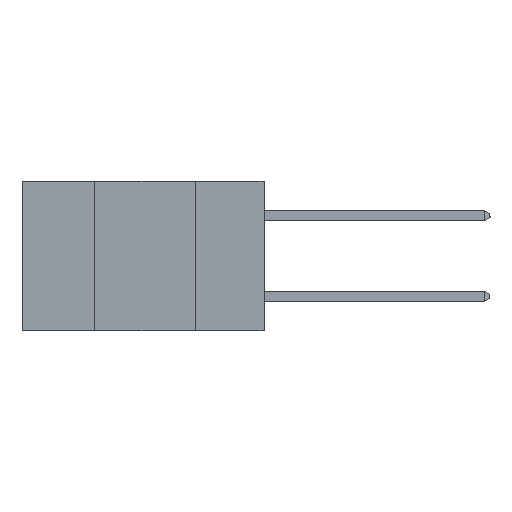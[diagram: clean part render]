
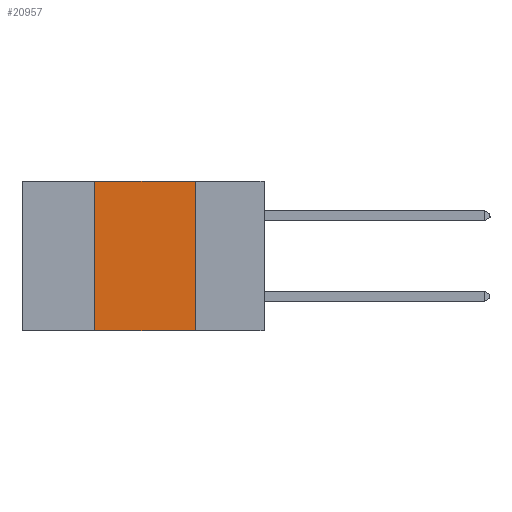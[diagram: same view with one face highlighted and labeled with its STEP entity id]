
A CAD part, left-side view. The second image highlights one B-rep face of the part: STEP entity #20957.
In plain terms, the highlighted planar face has unit normal (-1, 0, 0).
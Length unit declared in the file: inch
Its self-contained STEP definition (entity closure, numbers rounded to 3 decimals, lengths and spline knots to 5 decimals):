
#307 = VERTEX_POINT ( 'NONE', #8953 ) ;
#450 = ORIENTED_EDGE ( 'NONE', *, *, #4845, .F. ) ;
#1586 = AXIS2_PLACEMENT_3D ( 'NONE', #9550, #26071, #13766 ) ;
#1791 = LINE ( 'NONE', #19559, #22508 ) ;
#2050 = LINE ( 'NONE', #19369, #16722 ) ;
#4401 = FACE_OUTER_BOUND ( 'NONE', #11159, .T. ) ;
#4845 = EDGE_CURVE ( 'NONE', #18505, #307, #6566, .T. ) ;
#5902 = DIRECTION ( 'NONE',  ( 0., 0., 1. ) ) ;
#6032 = CARTESIAN_POINT ( 'NONE',  ( 0., 0.17, -0.37 ) ) ;
#6363 = CARTESIAN_POINT ( 'NONE',  ( 0., 0.42, -0.37 ) ) ;
#6566 = LINE ( 'NONE', #16216, #22430 ) ;
#8953 = CARTESIAN_POINT ( 'NONE',  ( 0., 0.42, 0. ) ) ;
#9463 = VECTOR ( 'NONE', #15052, 39.37008 ) ;
#9550 = CARTESIAN_POINT ( 'NONE',  ( 0., 0.6, 0. ) ) ;
#11159 = EDGE_LOOP ( 'NONE', ( #15808, #21858, #450, #11524 ) ) ;
#11524 = ORIENTED_EDGE ( 'NONE', *, *, #17926, .T. ) ;
#12792 = VERTEX_POINT ( 'NONE', #26674 ) ;
#12945 = CARTESIAN_POINT ( 'NONE',  ( 0., 0.6, -0.37 ) ) ;
#13123 = EDGE_CURVE ( 'NONE', #307, #12792, #2050, .T. ) ;
#13457 = DIRECTION ( 'NONE',  ( 0., 0., -1. ) ) ;
#13766 = DIRECTION ( 'NONE',  ( 0., 0., -1. ) ) ;
#15052 = DIRECTION ( 'NONE',  ( 0., -1., 0. ) ) ;
#15808 = ORIENTED_EDGE ( 'NONE', *, *, #21511, .F. ) ;
#16216 = CARTESIAN_POINT ( 'NONE',  ( 0., 0.42, 0. ) ) ;
#16645 = VERTEX_POINT ( 'NONE', #6032 ) ;
#16722 = VECTOR ( 'NONE', #25663, 39.37008 ) ;
#17926 = EDGE_CURVE ( 'NONE', #18505, #16645, #25303, .T. ) ;
#18505 = VERTEX_POINT ( 'NONE', #6363 ) ;
#19369 = CARTESIAN_POINT ( 'NONE',  ( 0., 0.6, 0. ) ) ;
#19559 = CARTESIAN_POINT ( 'NONE',  ( 0., 0.17, 0. ) ) ;
#20957 = ADVANCED_FACE ( 'NONE', ( #4401 ), #21932, .F. ) ;
#21511 = EDGE_CURVE ( 'NONE', #12792, #16645, #1791, .T. ) ;
#21858 = ORIENTED_EDGE ( 'NONE', *, *, #13123, .F. ) ;
#21932 = PLANE ( 'NONE',  #1586 ) ;
#22430 = VECTOR ( 'NONE', #5902, 39.37008 ) ;
#22508 = VECTOR ( 'NONE', #13457, 39.37008 ) ;
#25303 = LINE ( 'NONE', #12945, #9463 ) ;
#25663 = DIRECTION ( 'NONE',  ( 0., -1., 0. ) ) ;
#26071 = DIRECTION ( 'NONE',  ( 1., 0., 0. ) ) ;
#26674 = CARTESIAN_POINT ( 'NONE',  ( 0., 0.17, 0. ) ) ;
